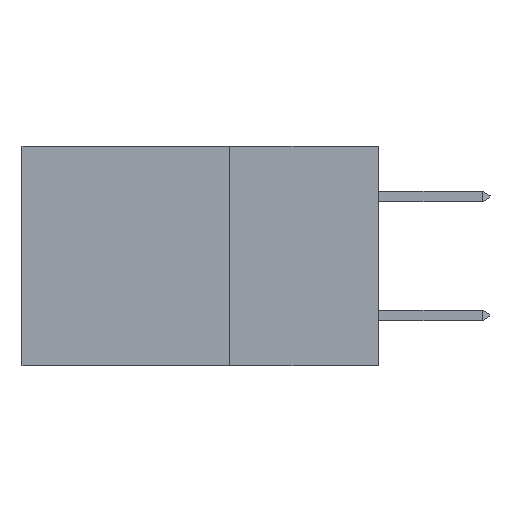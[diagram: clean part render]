
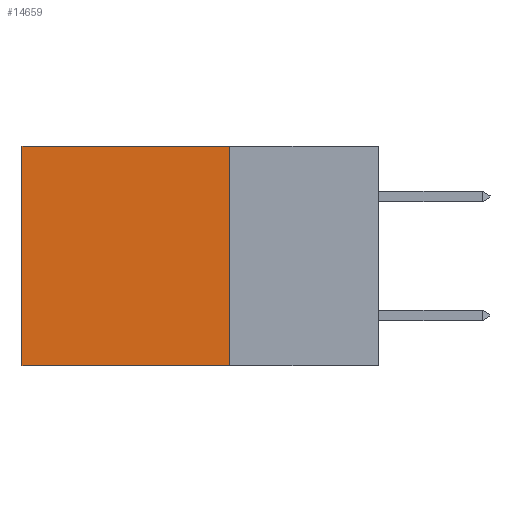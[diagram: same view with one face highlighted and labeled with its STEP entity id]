
A CAD part, left-side view. The second image highlights one B-rep face of the part: STEP entity #14659.
In plain terms, the highlighted planar face has unit normal (-1, 0, 0).
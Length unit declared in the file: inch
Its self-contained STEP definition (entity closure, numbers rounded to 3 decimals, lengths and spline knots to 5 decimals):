
#261 = DIRECTION ( 'NONE',  ( 0., 0., -1. ) ) ;
#763 = FACE_OUTER_BOUND ( 'NONE', #4959, .T. ) ;
#1000 = DIRECTION ( 'NONE',  ( 1., 0., 0. ) ) ;
#1218 = CARTESIAN_POINT ( 'NONE',  ( 0.2615, 0.6, -0.37 ) ) ;
#1602 = LINE ( 'NONE', #9981, #7888 ) ;
#2192 = CARTESIAN_POINT ( 'NONE',  ( 0.2615, 0.25, -0.37 ) ) ;
#2346 = LINE ( 'NONE', #14171, #7725 ) ;
#2444 = ORIENTED_EDGE ( 'NONE', *, *, #14598, .T. ) ;
#3457 = DIRECTION ( 'NONE',  ( 0., 0., -1. ) ) ;
#4171 = DIRECTION ( 'NONE',  ( 0., 1., 0. ) ) ;
#4309 = LINE ( 'NONE', #11367, #8643 ) ;
#4524 = EDGE_CURVE ( 'NONE', #10324, #12228, #4606, .T. ) ;
#4606 = LINE ( 'NONE', #7120, #13783 ) ;
#4959 = EDGE_LOOP ( 'NONE', ( #7233, #15174, #8258, #2444 ) ) ;
#5176 = CARTESIAN_POINT ( 'NONE',  ( 0.2615, 0.25, -0.37 ) ) ;
#7120 = CARTESIAN_POINT ( 'NONE',  ( 0.2615, 0.6, -0.37 ) ) ;
#7233 = ORIENTED_EDGE ( 'NONE', *, *, #4524, .T. ) ;
#7725 = VECTOR ( 'NONE', #14018, 39.37008 ) ;
#7888 = VECTOR ( 'NONE', #261, 39.37008 ) ;
#8258 = ORIENTED_EDGE ( 'NONE', *, *, #10964, .F. ) ;
#8276 = VERTEX_POINT ( 'NONE', #9486 ) ;
#8643 = VECTOR ( 'NONE', #4171, 39.37008 ) ;
#9368 = DIRECTION ( 'NONE',  ( 0., 0., -1. ) ) ;
#9486 = CARTESIAN_POINT ( 'NONE',  ( 0.2615, 0.25, 0. ) ) ;
#9981 = CARTESIAN_POINT ( 'NONE',  ( 0.2615, 0.25, -0.37 ) ) ;
#10324 = VERTEX_POINT ( 'NONE', #12857 ) ;
#10327 = PLANE ( 'NONE',  #13229 ) ;
#10964 = EDGE_CURVE ( 'NONE', #8276, #11340, #1602, .T. ) ;
#11340 = VERTEX_POINT ( 'NONE', #5176 ) ;
#11367 = CARTESIAN_POINT ( 'NONE',  ( 0.2615, 0.25, -0.37 ) ) ;
#11410 = EDGE_CURVE ( 'NONE', #11340, #12228, #4309, .T. ) ;
#12228 = VERTEX_POINT ( 'NONE', #1218 ) ;
#12857 = CARTESIAN_POINT ( 'NONE',  ( 0.2615, 0.6, 0. ) ) ;
#13229 = AXIS2_PLACEMENT_3D ( 'NONE', #2192, #1000, #3457 ) ;
#13783 = VECTOR ( 'NONE', #9368, 39.37008 ) ;
#14018 = DIRECTION ( 'NONE',  ( 0., 1., 0. ) ) ;
#14171 = CARTESIAN_POINT ( 'NONE',  ( 0.2615, 0.25, 0. ) ) ;
#14598 = EDGE_CURVE ( 'NONE', #8276, #10324, #2346, .T. ) ;
#14659 = ADVANCED_FACE ( 'NONE', ( #763 ), #10327, .F. ) ;
#15174 = ORIENTED_EDGE ( 'NONE', *, *, #11410, .F. ) ;
